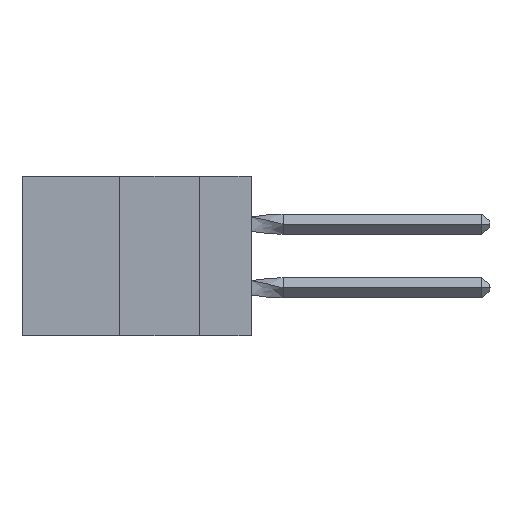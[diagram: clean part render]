
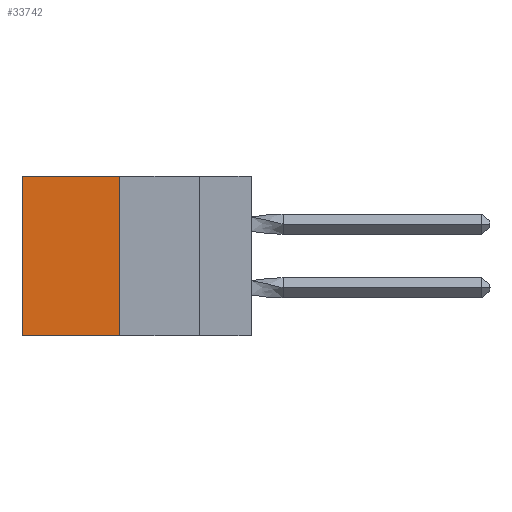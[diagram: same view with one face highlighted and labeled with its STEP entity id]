
A CAD part, left-side view. The second image highlights one B-rep face of the part: STEP entity #33742.
In plain terms, the highlighted planar face has unit normal (-1, 0, 0).
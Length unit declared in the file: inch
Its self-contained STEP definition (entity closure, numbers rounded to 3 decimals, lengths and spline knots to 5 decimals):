
#706 = CARTESIAN_POINT ( 'NONE',  ( 0.305, 0.413, 0. ) ) ;
#1715 = DIRECTION ( 'NONE',  ( 0., 1., 0. ) ) ;
#2341 = CARTESIAN_POINT ( 'NONE',  ( 0.305, 0.72, 0. ) ) ;
#2644 = EDGE_CURVE ( 'NONE', #33314, #26451, #23648, .T. ) ;
#2750 = DIRECTION ( 'NONE',  ( 0., 0., -1. ) ) ;
#3092 = VERTEX_POINT ( 'NONE', #2341 ) ;
#5370 = CARTESIAN_POINT ( 'NONE',  ( 0.305, 0.413, -0.5 ) ) ;
#8591 = LINE ( 'NONE', #5370, #21927 ) ;
#8715 = DIRECTION ( 'NONE',  ( 1., 0., 0. ) ) ;
#9346 = VECTOR ( 'NONE', #1715, 39.37008 ) ;
#10295 = FACE_OUTER_BOUND ( 'NONE', #11438, .T. ) ;
#10328 = VECTOR ( 'NONE', #22465, 39.37008 ) ;
#10785 = ORIENTED_EDGE ( 'NONE', *, *, #37421, .T. ) ;
#11438 = EDGE_LOOP ( 'NONE', ( #10785, #37847, #14481, #39427 ) ) ;
#14481 = ORIENTED_EDGE ( 'NONE', *, *, #2644, .F. ) ;
#15932 = LINE ( 'NONE', #19022, #35167 ) ;
#18925 = VERTEX_POINT ( 'NONE', #36483 ) ;
#19022 = CARTESIAN_POINT ( 'NONE',  ( 0.305, 0.72, -0.5 ) ) ;
#19293 = EDGE_CURVE ( 'NONE', #26451, #18925, #8591, .T. ) ;
#21775 = DIRECTION ( 'NONE',  ( 0., 0., -1. ) ) ;
#21927 = VECTOR ( 'NONE', #40087, 39.37008 ) ;
#22465 = DIRECTION ( 'NONE',  ( 0., 0., -1. ) ) ;
#23648 = LINE ( 'NONE', #32952, #10328 ) ;
#24035 = CARTESIAN_POINT ( 'NONE',  ( 0.305, 0.413, -0.5 ) ) ;
#26451 = VERTEX_POINT ( 'NONE', #24035 ) ;
#27100 = LINE ( 'NONE', #40008, #9346 ) ;
#27480 = PLANE ( 'NONE',  #40901 ) ;
#32952 = CARTESIAN_POINT ( 'NONE',  ( 0.305, 0.413, -0.5 ) ) ;
#33314 = VERTEX_POINT ( 'NONE', #706 ) ;
#33742 = ADVANCED_FACE ( 'NONE', ( #10295 ), #27480, .F. ) ;
#35167 = VECTOR ( 'NONE', #21775, 39.37008 ) ;
#36483 = CARTESIAN_POINT ( 'NONE',  ( 0.305, 0.72, -0.5 ) ) ;
#37025 = CARTESIAN_POINT ( 'NONE',  ( 0.305, 0.413, -0.5 ) ) ;
#37421 = EDGE_CURVE ( 'NONE', #3092, #18925, #15932, .T. ) ;
#37847 = ORIENTED_EDGE ( 'NONE', *, *, #19293, .F. ) ;
#39427 = ORIENTED_EDGE ( 'NONE', *, *, #39655, .T. ) ;
#39655 = EDGE_CURVE ( 'NONE', #33314, #3092, #27100, .T. ) ;
#40008 = CARTESIAN_POINT ( 'NONE',  ( 0.305, 0.413, 0. ) ) ;
#40087 = DIRECTION ( 'NONE',  ( 0., 1., 0. ) ) ;
#40901 = AXIS2_PLACEMENT_3D ( 'NONE', #37025, #8715, #2750 ) ;
